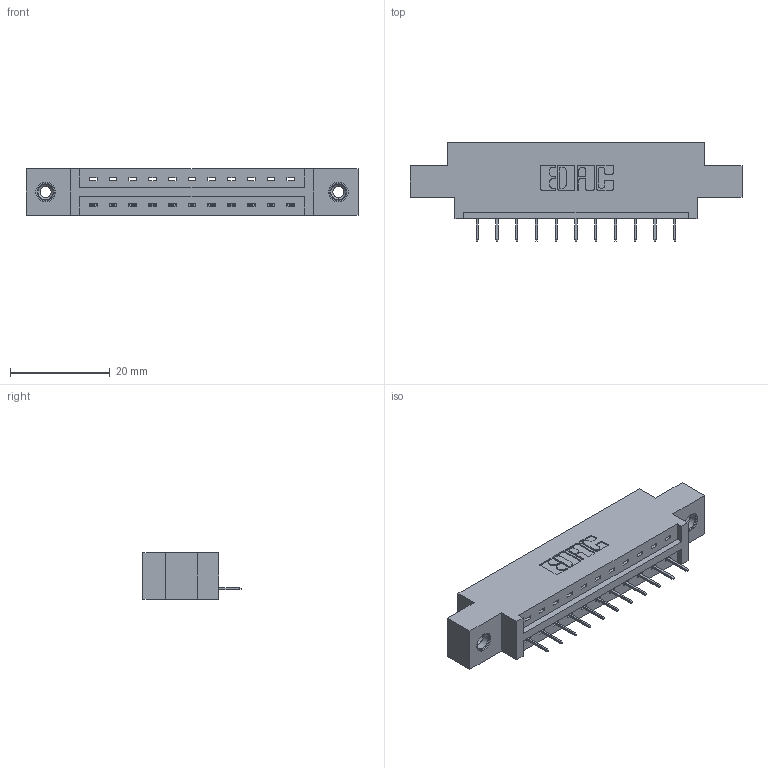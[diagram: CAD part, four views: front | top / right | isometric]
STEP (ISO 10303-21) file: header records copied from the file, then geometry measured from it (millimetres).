
FILE_DESCRIPTION (( 'STEP AP203' ), '1' );
FILE_NAME ('337-011-524-608.STEP', '2018-08-04T01:25:38', ( '' ), ( '' ), 'SwSTEP 2.0', 'SolidWorks 2016', '' );
FILE_SCHEMA (( 'CONFIG_CONTROL_DESIGN' ));
Length unit declared in the file: inch
Products named in the file (4): 337-011-524-608; 337 Part_0.170 Offset - 0.156 Dia-TI; 345-292-001_345-293-124; 345-250-001_345-250-003-102
Assembly tree (14 placements, depth 2):
  337-011-524-608
    337 Part_0.170 Offset - 0.156 Dia-TI
    345-292-001_345-293-124  x11
    345-250-001_345-250-003-102  x2
Bounding box: 66.6 x 19.69 x 9.4 mm (x, y, z)
Volume: 6366.4 mm3; surface area: 6380 mm2
Topology: 14 solids, 14 shells, 904 faces, 2571 edges, 1662 vertices
Faces by surface type: plane 678, cylinder 210, cone 12, torus 4
Entity records: 13578 total; most frequent: CARTESIAN_POINT 2342, ORIENTED_EDGE 2282, DIRECTION 2069, EDGE_CURVE 1141, VECTOR 997, LINE 997, VERTEX_POINT 752, AXIS2_PLACEMENT_3D 536
